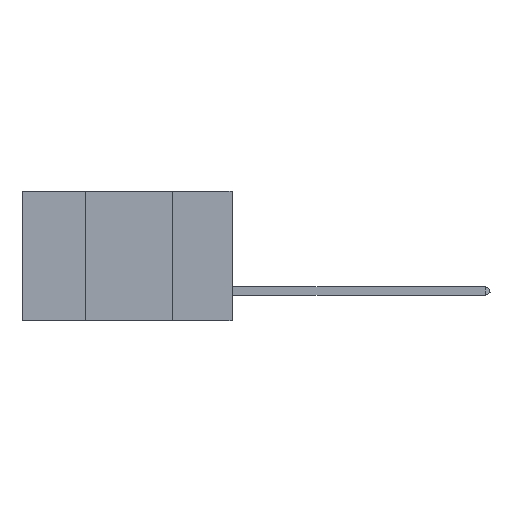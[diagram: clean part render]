
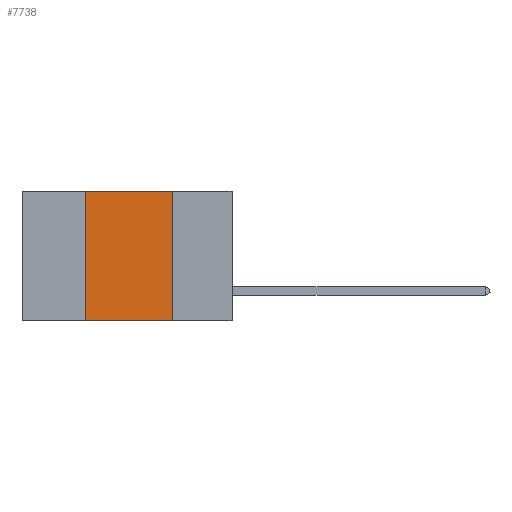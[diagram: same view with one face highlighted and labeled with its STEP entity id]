
A CAD part, left-side view. The second image highlights one B-rep face of the part: STEP entity #7738.
In plain terms, the highlighted planar face has unit normal (-1, 0, 0).
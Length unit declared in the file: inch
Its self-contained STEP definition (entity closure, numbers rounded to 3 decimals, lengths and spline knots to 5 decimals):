
#221 = CARTESIAN_POINT ( 'NONE',  ( 0., 0.6, 0. ) ) ;
#1073 = ORIENTED_EDGE ( 'NONE', *, *, #2816, .F. ) ;
#1470 = DIRECTION ( 'NONE',  ( 0., -1., 0. ) ) ;
#2704 = DIRECTION ( 'NONE',  ( 1., 0., 0. ) ) ;
#2816 = EDGE_CURVE ( 'NONE', #31990, #6277, #5484, .T. ) ;
#3366 = VERTEX_POINT ( 'NONE', #8107 ) ;
#5484 = LINE ( 'NONE', #9979, #24971 ) ;
#6277 = VERTEX_POINT ( 'NONE', #19971 ) ;
#6891 = VECTOR ( 'NONE', #1470, 39.37008 ) ;
#7738 = ADVANCED_FACE ( 'NONE', ( #30918 ), #18137, .F. ) ;
#8107 = CARTESIAN_POINT ( 'NONE',  ( 0., 0.42, 0. ) ) ;
#9471 = LINE ( 'NONE', #24733, #14832 ) ;
#9979 = CARTESIAN_POINT ( 'NONE',  ( 0., 0.17, 0. ) ) ;
#10763 = LINE ( 'NONE', #13241, #21391 ) ;
#10820 = VERTEX_POINT ( 'NONE', #20509 ) ;
#11527 = ORIENTED_EDGE ( 'NONE', *, *, #14559, .F. ) ;
#11993 = ORIENTED_EDGE ( 'NONE', *, *, #29978, .T. ) ;
#13241 = CARTESIAN_POINT ( 'NONE',  ( 0., 0.42, 0. ) ) ;
#14559 = EDGE_CURVE ( 'NONE', #10820, #3366, #10763, .T. ) ;
#14832 = VECTOR ( 'NONE', #22424, 39.37008 ) ;
#17658 = ORIENTED_EDGE ( 'NONE', *, *, #23627, .F. ) ;
#18137 = PLANE ( 'NONE',  #28976 ) ;
#19971 = CARTESIAN_POINT ( 'NONE',  ( 0., 0.17, -0.37 ) ) ;
#20509 = CARTESIAN_POINT ( 'NONE',  ( 0., 0.42, -0.37 ) ) ;
#21391 = VECTOR ( 'NONE', #23196, 39.37008 ) ;
#22050 = LINE ( 'NONE', #26538, #6891 ) ;
#22424 = DIRECTION ( 'NONE',  ( 0., -1., 0. ) ) ;
#23196 = DIRECTION ( 'NONE',  ( 0., 0., 1. ) ) ;
#23627 = EDGE_CURVE ( 'NONE', #3366, #31990, #22050, .T. ) ;
#24604 = EDGE_LOOP ( 'NONE', ( #1073, #17658, #11527, #11993 ) ) ;
#24733 = CARTESIAN_POINT ( 'NONE',  ( 0., 0.6, -0.37 ) ) ;
#24971 = VECTOR ( 'NONE', #25723, 39.37008 ) ;
#25723 = DIRECTION ( 'NONE',  ( 0., 0., -1. ) ) ;
#25831 = CARTESIAN_POINT ( 'NONE',  ( 0., 0.17, 0. ) ) ;
#26538 = CARTESIAN_POINT ( 'NONE',  ( 0., 0.6, 0. ) ) ;
#28430 = DIRECTION ( 'NONE',  ( 0., 0., -1. ) ) ;
#28976 = AXIS2_PLACEMENT_3D ( 'NONE', #221, #2704, #28430 ) ;
#29978 = EDGE_CURVE ( 'NONE', #10820, #6277, #9471, .T. ) ;
#30918 = FACE_OUTER_BOUND ( 'NONE', #24604, .T. ) ;
#31990 = VERTEX_POINT ( 'NONE', #25831 ) ;
